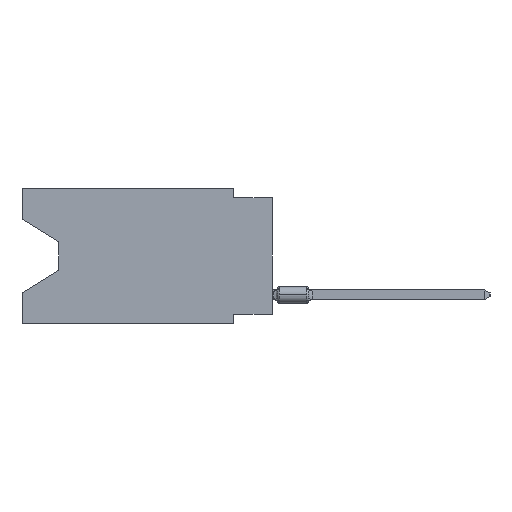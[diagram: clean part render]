
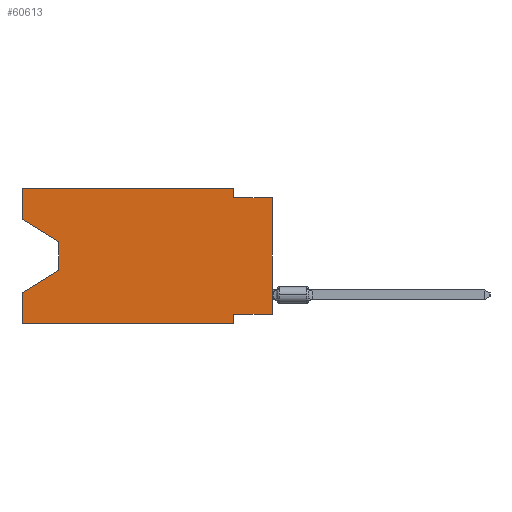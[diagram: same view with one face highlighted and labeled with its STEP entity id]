
A CAD part, left-side view. The second image highlights one B-rep face of the part: STEP entity #60613.
In plain terms, the highlighted planar face has unit normal (-1, 0, 0).
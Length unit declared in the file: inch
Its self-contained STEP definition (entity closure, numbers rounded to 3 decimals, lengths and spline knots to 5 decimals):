
#255 = CARTESIAN_POINT ( 'NONE',  ( 0., 0.645, 0. ) ) ;
#284 = CARTESIAN_POINT ( 'NONE',  ( 0., 0.645, 0. ) ) ;
#393 = CARTESIAN_POINT ( 'NONE',  ( 0., 0., -0.325 ) ) ;
#1928 = ORIENTED_EDGE ( 'NONE', *, *, #22801, .T. ) ;
#2289 = LINE ( 'NONE', #8106, #25507 ) ;
#2517 = EDGE_CURVE ( 'NONE', #41909, #9970, #46252, .T. ) ;
#3198 = ORIENTED_EDGE ( 'NONE', *, *, #58061, .F. ) ;
#3965 = CARTESIAN_POINT ( 'NONE',  ( 0., 0.1, 0. ) ) ;
#4427 = ORIENTED_EDGE ( 'NONE', *, *, #48404, .F. ) ;
#4992 = DIRECTION ( 'NONE',  ( 0., -0.855, -0.519 ) ) ;
#5243 = CARTESIAN_POINT ( 'NONE',  ( 0., 0.55, -0.138 ) ) ;
#5446 = VERTEX_POINT ( 'NONE', #393 ) ;
#6050 = EDGE_CURVE ( 'NONE', #37968, #6500, #57831, .T. ) ;
#6500 = VERTEX_POINT ( 'NONE', #284 ) ;
#6511 = DIRECTION ( 'NONE',  ( 0., 0., 1. ) ) ;
#6592 = LINE ( 'NONE', #5243, #57231 ) ;
#8106 = CARTESIAN_POINT ( 'NONE',  ( 0., 0., -0.325 ) ) ;
#8948 = VECTOR ( 'NONE', #60065, 39.37008 ) ;
#9136 = CARTESIAN_POINT ( 'NONE',  ( 0., 0., -0.025 ) ) ;
#9586 = CARTESIAN_POINT ( 'NONE',  ( 0., 0.645, -0.35 ) ) ;
#9970 = VERTEX_POINT ( 'NONE', #17848 ) ;
#11367 = VERTEX_POINT ( 'NONE', #63793 ) ;
#12419 = EDGE_CURVE ( 'NONE', #37968, #50323, #60781, .T. ) ;
#13202 = CARTESIAN_POINT ( 'NONE',  ( 0., 0., 0. ) ) ;
#14910 = VECTOR ( 'NONE', #16003, 39.37008 ) ;
#15137 = LINE ( 'NONE', #45628, #47035 ) ;
#16003 = DIRECTION ( 'NONE',  ( 0., 0., 1. ) ) ;
#16666 = CARTESIAN_POINT ( 'NONE',  ( 0., 0.1, 0. ) ) ;
#17848 = CARTESIAN_POINT ( 'NONE',  ( 0., 0.645, -0.26975 ) ) ;
#18005 = CARTESIAN_POINT ( 'NONE',  ( 0., 0.645, 0. ) ) ;
#18713 = DIRECTION ( 'NONE',  ( 0., 1., 0. ) ) ;
#18735 = LINE ( 'NONE', #9136, #61071 ) ;
#19826 = ORIENTED_EDGE ( 'NONE', *, *, #2517, .T. ) ;
#19913 = DIRECTION ( 'NONE',  ( 0., 0.855, -0.519 ) ) ;
#20721 = ORIENTED_EDGE ( 'NONE', *, *, #58045, .F. ) ;
#21122 = LINE ( 'NONE', #16666, #50970 ) ;
#22801 = EDGE_CURVE ( 'NONE', #50323, #41909, #6592, .T. ) ;
#23867 = DIRECTION ( 'NONE',  ( 0., -1., 0. ) ) ;
#24154 = VECTOR ( 'NONE', #30783, 39.37008 ) ;
#24374 = CARTESIAN_POINT ( 'NONE',  ( 0., 0.1, -0.35 ) ) ;
#25389 = ORIENTED_EDGE ( 'NONE', *, *, #12419, .T. ) ;
#25483 = DIRECTION ( 'NONE',  ( 0., 0., -1. ) ) ;
#25507 = VECTOR ( 'NONE', #18713, 39.37008 ) ;
#26095 = DIRECTION ( 'NONE',  ( 0., 0., -1. ) ) ;
#26577 = CARTESIAN_POINT ( 'NONE',  ( 0., 0.1, -0.325 ) ) ;
#27400 = VECTOR ( 'NONE', #19913, 39.37008 ) ;
#28327 = EDGE_CURVE ( 'NONE', #42111, #46536, #18735, .T. ) ;
#29653 = CARTESIAN_POINT ( 'NONE',  ( 0., 0.645, -0.08025 ) ) ;
#30002 = CARTESIAN_POINT ( 'NONE',  ( 0., 0.645, -0.08025 ) ) ;
#30317 = VERTEX_POINT ( 'NONE', #3965 ) ;
#30783 = DIRECTION ( 'NONE',  ( 0., -1., 0. ) ) ;
#32111 = EDGE_CURVE ( 'NONE', #66415, #51531, #15137, .T. ) ;
#32677 = ORIENTED_EDGE ( 'NONE', *, *, #28327, .F. ) ;
#33172 = CARTESIAN_POINT ( 'NONE',  ( 0., 0., -0.025 ) ) ;
#33470 = EDGE_CURVE ( 'NONE', #5446, #46536, #64862, .T. ) ;
#34677 = ORIENTED_EDGE ( 'NONE', *, *, #33470, .T. ) ;
#34758 = DIRECTION ( 'NONE',  ( 1., 0., 0. ) ) ;
#35483 = ORIENTED_EDGE ( 'NONE', *, *, #6050, .F. ) ;
#35753 = CARTESIAN_POINT ( 'NONE',  ( 0., 0.645, 0. ) ) ;
#36003 = DIRECTION ( 'NONE',  ( 0., 0., -1. ) ) ;
#36283 = CARTESIAN_POINT ( 'NONE',  ( 0., 0.645, 0. ) ) ;
#36660 = CARTESIAN_POINT ( 'NONE',  ( 0., 0.55, -0.212 ) ) ;
#37593 = ORIENTED_EDGE ( 'NONE', *, *, #45093, .T. ) ;
#37968 = VERTEX_POINT ( 'NONE', #30002 ) ;
#40147 = AXIS2_PLACEMENT_3D ( 'NONE', #35753, #34758, #25483 ) ;
#40872 = CARTESIAN_POINT ( 'NONE',  ( 0., 0.55, -0.212 ) ) ;
#41909 = VERTEX_POINT ( 'NONE', #40872 ) ;
#42033 = LINE ( 'NONE', #255, #14910 ) ;
#42111 = VERTEX_POINT ( 'NONE', #60281 ) ;
#44574 = ORIENTED_EDGE ( 'NONE', *, *, #32111, .F. ) ;
#45093 = EDGE_CURVE ( 'NONE', #11367, #51531, #67057, .T. ) ;
#45542 = ORIENTED_EDGE ( 'NONE', *, *, #60572, .F. ) ;
#45628 = CARTESIAN_POINT ( 'NONE',  ( 0., 0.1, -0.35 ) ) ;
#46252 = LINE ( 'NONE', #36660, #27400 ) ;
#46536 = VERTEX_POINT ( 'NONE', #33172 ) ;
#46799 = DIRECTION ( 'NONE',  ( 0., 0., -1. ) ) ;
#47035 = VECTOR ( 'NONE', #36003, 39.37008 ) ;
#48404 = EDGE_CURVE ( 'NONE', #5446, #66415, #2289, .T. ) ;
#48808 = PLANE ( 'NONE',  #40147 ) ;
#50323 = VERTEX_POINT ( 'NONE', #65423 ) ;
#50970 = VECTOR ( 'NONE', #46799, 39.37008 ) ;
#51531 = VERTEX_POINT ( 'NONE', #24374 ) ;
#53809 = VECTOR ( 'NONE', #6511, 39.37008 ) ;
#54275 = DIRECTION ( 'NONE',  ( 0., -1., 0. ) ) ;
#57231 = VECTOR ( 'NONE', #26095, 39.37008 ) ;
#57388 = VECTOR ( 'NONE', #4992, 39.37008 ) ;
#57831 = LINE ( 'NONE', #36283, #53809 ) ;
#58045 = EDGE_CURVE ( 'NONE', #30317, #42111, #21122, .T. ) ;
#58061 = EDGE_CURVE ( 'NONE', #11367, #9970, #42033, .T. ) ;
#58712 = VECTOR ( 'NONE', #54275, 39.37008 ) ;
#59395 = LINE ( 'NONE', #18005, #58712 ) ;
#59734 = FACE_OUTER_BOUND ( 'NONE', #61146, .T. ) ;
#60065 = DIRECTION ( 'NONE',  ( 0., 0., 1. ) ) ;
#60281 = CARTESIAN_POINT ( 'NONE',  ( 0., 0.1, -0.025 ) ) ;
#60572 = EDGE_CURVE ( 'NONE', #6500, #30317, #59395, .T. ) ;
#60613 = ADVANCED_FACE ( 'NONE', ( #59734 ), #48808, .F. ) ;
#60781 = LINE ( 'NONE', #29653, #57388 ) ;
#61071 = VECTOR ( 'NONE', #23867, 39.37008 ) ;
#61146 = EDGE_LOOP ( 'NONE', ( #25389, #1928, #19826, #3198, #37593, #44574, #4427, #34677, #32677, #20721, #45542, #35483 ) ) ;
#63793 = CARTESIAN_POINT ( 'NONE',  ( 0., 0.645, -0.35 ) ) ;
#64862 = LINE ( 'NONE', #13202, #8948 ) ;
#65423 = CARTESIAN_POINT ( 'NONE',  ( 0., 0.55, -0.138 ) ) ;
#66415 = VERTEX_POINT ( 'NONE', #26577 ) ;
#67057 = LINE ( 'NONE', #9586, #24154 ) ;
